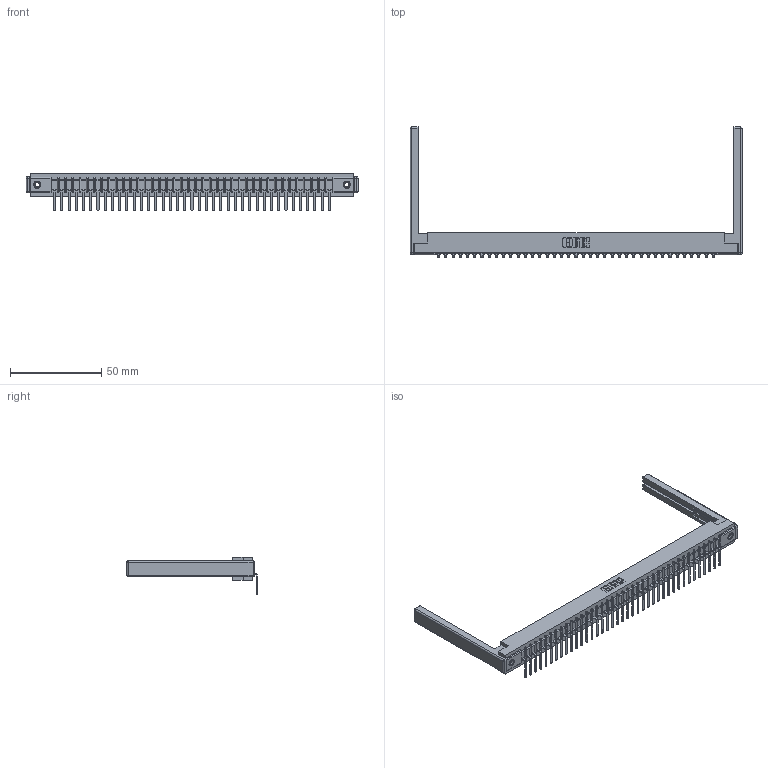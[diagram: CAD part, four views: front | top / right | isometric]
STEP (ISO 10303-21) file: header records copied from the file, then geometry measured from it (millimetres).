
FILE_DESCRIPTION (( 'STEP AP203' ), '1' );
FILE_NAME ('357-039-457-168.STEP', '2020-10-03T04:45:10', ( '' ), ( '' ), 'SwSTEP 2.0', 'SolidWorks 2020', '' );
FILE_SCHEMA (( 'CONFIG_CONTROL_DESIGN' ));
Length unit declared in the file: inch
Products named in the file (5): 307 Part_.156 Dia Mounting Holes; 307-220-068; 345-250-001_345-250-001-102; 357-039-457-168; 307-290-002_557
Assembly tree (44 placements, depth 2):
  357-039-457-168
    307 Part_.156 Dia Mounting Holes
    307-290-002_557  x39
    307-220-068  x2
    345-250-001_345-250-001-102  x2
Bounding box: 181.97 x 71.29 x 20.66 mm (x, y, z)
Volume: 23933.1 mm3; surface area: 29167.7 mm2
Topology: 44 solids, 44 shells, 3354 faces, 10229 edges, 6690 vertices
Faces by surface type: plane 1991, cylinder 1259, sphere 88, cone 12, torus 4
Entity records: 37417 total; most frequent: CARTESIAN_POINT 6277, ORIENTED_EDGE 6256, DIRECTION 6118, EDGE_CURVE 3128, VECTOR 2392, LINE 2392, VERTEX_POINT 2022, AXIS2_PLACEMENT_3D 1863
